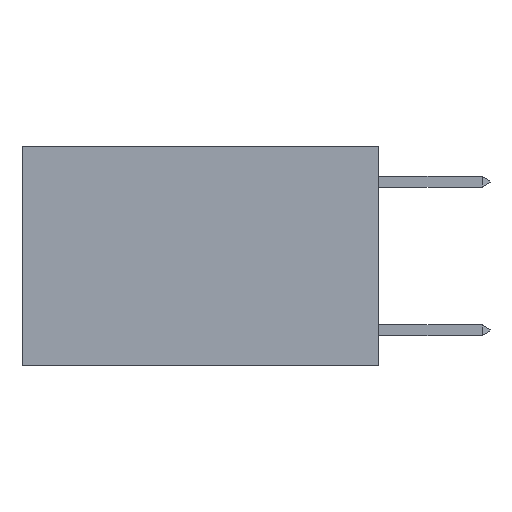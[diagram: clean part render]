
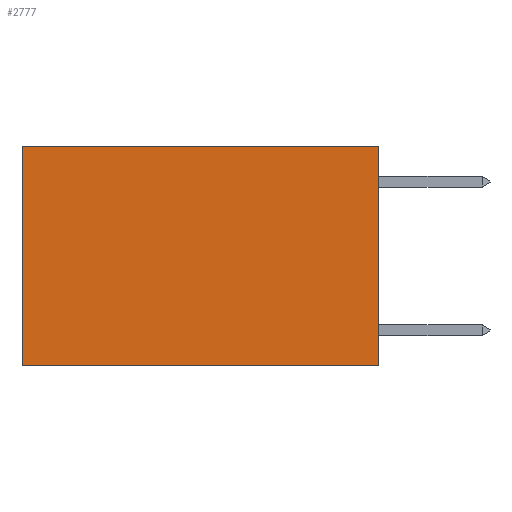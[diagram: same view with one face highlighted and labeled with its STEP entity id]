
A CAD part, left-side view. The second image highlights one B-rep face of the part: STEP entity #2777.
In plain terms, the highlighted planar face has unit normal (-1, 0, 0).
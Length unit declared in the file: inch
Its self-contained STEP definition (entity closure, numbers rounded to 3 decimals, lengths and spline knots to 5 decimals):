
#775 = DIRECTION ( 'NONE',  ( 0., 0., -1. ) ) ;
#1402 = CARTESIAN_POINT ( 'NONE',  ( 0.2625, 0., -0.37 ) ) ;
#1475 = AXIS2_PLACEMENT_3D ( 'NONE', #3577, #9551, #13962 ) ;
#2045 = EDGE_LOOP ( 'NONE', ( #11562, #6450, #3436, #7797 ) ) ;
#2512 = LINE ( 'NONE', #5650, #11537 ) ;
#2777 = ADVANCED_FACE ( 'NONE', ( #9227 ), #10252, .F. ) ;
#2866 = EDGE_CURVE ( 'NONE', #2872, #9337, #12021, .T. ) ;
#2872 = VERTEX_POINT ( 'NONE', #4199 ) ;
#3032 = CARTESIAN_POINT ( 'NONE',  ( 0.2625, 0., 0. ) ) ;
#3436 = ORIENTED_EDGE ( 'NONE', *, *, #2866, .F. ) ;
#3577 = CARTESIAN_POINT ( 'NONE',  ( 0.2625, 0., 0. ) ) ;
#4199 = CARTESIAN_POINT ( 'NONE',  ( 0.2625, 0., 0. ) ) ;
#4444 = VERTEX_POINT ( 'NONE', #7715 ) ;
#5042 = DIRECTION ( 'NONE',  ( 0., 1., 0. ) ) ;
#5650 = CARTESIAN_POINT ( 'NONE',  ( 0.2625, 0.6, 0. ) ) ;
#6212 = CARTESIAN_POINT ( 'NONE',  ( 0.2625, 0., 0. ) ) ;
#6450 = ORIENTED_EDGE ( 'NONE', *, *, #10464, .F. ) ;
#7715 = CARTESIAN_POINT ( 'NONE',  ( 0.2625, 0.6, 0. ) ) ;
#7797 = ORIENTED_EDGE ( 'NONE', *, *, #14061, .T. ) ;
#8581 = VECTOR ( 'NONE', #10493, 39.37008 ) ;
#9227 = FACE_OUTER_BOUND ( 'NONE', #2045, .T. ) ;
#9337 = VERTEX_POINT ( 'NONE', #1402 ) ;
#9551 = DIRECTION ( 'NONE',  ( 1., 0., 0. ) ) ;
#9929 = VECTOR ( 'NONE', #5042, 39.37008 ) ;
#9944 = EDGE_CURVE ( 'NONE', #4444, #12936, #2512, .T. ) ;
#10017 = CARTESIAN_POINT ( 'NONE',  ( 0.2625, 0.6, -0.37 ) ) ;
#10252 = PLANE ( 'NONE',  #1475 ) ;
#10464 = EDGE_CURVE ( 'NONE', #9337, #12936, #11468, .T. ) ;
#10493 = DIRECTION ( 'NONE',  ( 0., 1., 0. ) ) ;
#11468 = LINE ( 'NONE', #12484, #9929 ) ;
#11537 = VECTOR ( 'NONE', #13516, 39.37008 ) ;
#11562 = ORIENTED_EDGE ( 'NONE', *, *, #9944, .T. ) ;
#11669 = VECTOR ( 'NONE', #775, 39.37008 ) ;
#11850 = LINE ( 'NONE', #6212, #8581 ) ;
#12021 = LINE ( 'NONE', #3032, #11669 ) ;
#12484 = CARTESIAN_POINT ( 'NONE',  ( 0.2625, 0., -0.37 ) ) ;
#12936 = VERTEX_POINT ( 'NONE', #10017 ) ;
#13516 = DIRECTION ( 'NONE',  ( 0., 0., -1. ) ) ;
#13962 = DIRECTION ( 'NONE',  ( 0., 0., -1. ) ) ;
#14061 = EDGE_CURVE ( 'NONE', #2872, #4444, #11850, .T. ) ;
